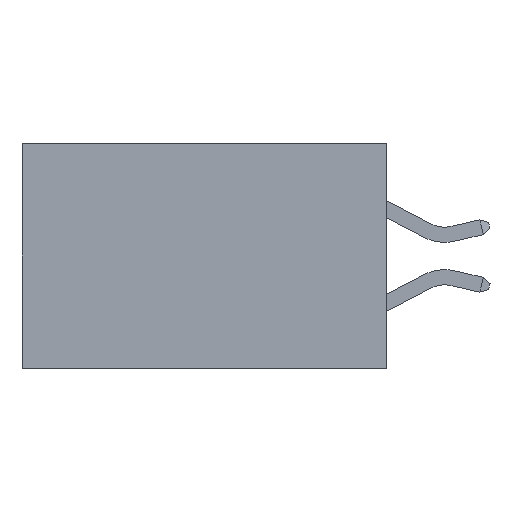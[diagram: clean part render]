
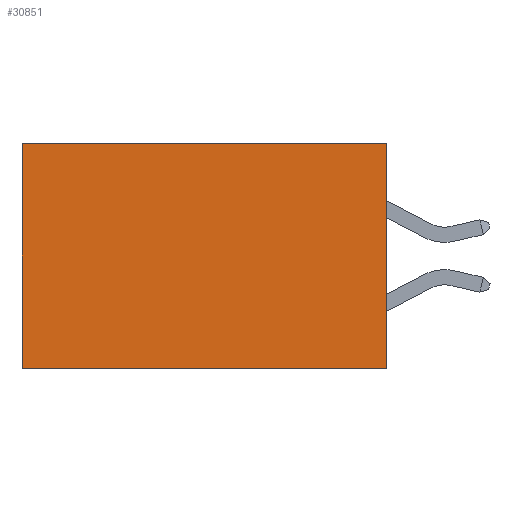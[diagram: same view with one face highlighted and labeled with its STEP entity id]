
A CAD part, left-side view. The second image highlights one B-rep face of the part: STEP entity #30851.
In plain terms, the highlighted planar face has unit normal (-1, 0, 0).
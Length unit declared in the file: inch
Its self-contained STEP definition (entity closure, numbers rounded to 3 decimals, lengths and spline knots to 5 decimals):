
#298 = DIRECTION ( 'NONE',  ( 0., 1., 0. ) ) ;
#1716 = LINE ( 'NONE', #13113, #17820 ) ;
#1743 = VERTEX_POINT ( 'NONE', #19567 ) ;
#1802 = FACE_OUTER_BOUND ( 'NONE', #3720, .T. ) ;
#3399 = CARTESIAN_POINT ( 'NONE',  ( 0.298, 0., 0. ) ) ;
#3720 = EDGE_LOOP ( 'NONE', ( #17352, #19211, #10265, #28102 ) ) ;
#4675 = VECTOR ( 'NONE', #298, 39.37008 ) ;
#5066 = EDGE_CURVE ( 'NONE', #1743, #6829, #15802, .T. ) ;
#5516 = CARTESIAN_POINT ( 'NONE',  ( 0.298, 0., 0. ) ) ;
#5920 = VERTEX_POINT ( 'NONE', #29874 ) ;
#6471 = VECTOR ( 'NONE', #28961, 39.37008 ) ;
#6829 = VERTEX_POINT ( 'NONE', #20515 ) ;
#10265 = ORIENTED_EDGE ( 'NONE', *, *, #27786, .F. ) ;
#10285 = LINE ( 'NONE', #19204, #6471 ) ;
#11252 = CARTESIAN_POINT ( 'NONE',  ( 0.298, 0., -0.37 ) ) ;
#12782 = PLANE ( 'NONE',  #29883 ) ;
#13113 = CARTESIAN_POINT ( 'NONE',  ( 0.298, 0., 0. ) ) ;
#13757 = VERTEX_POINT ( 'NONE', #11252 ) ;
#15802 = LINE ( 'NONE', #5516, #29763 ) ;
#17352 = ORIENTED_EDGE ( 'NONE', *, *, #29684, .T. ) ;
#17820 = VECTOR ( 'NONE', #20658, 39.37008 ) ;
#19204 = CARTESIAN_POINT ( 'NONE',  ( 0.298, 0.6, 0. ) ) ;
#19211 = ORIENTED_EDGE ( 'NONE', *, *, #22162, .F. ) ;
#19567 = CARTESIAN_POINT ( 'NONE',  ( 0.298, 0., 0. ) ) ;
#19731 = CARTESIAN_POINT ( 'NONE',  ( 0.298, 0., -0.37 ) ) ;
#20515 = CARTESIAN_POINT ( 'NONE',  ( 0.298, 0.6, 0. ) ) ;
#20658 = DIRECTION ( 'NONE',  ( 0., 0., -1. ) ) ;
#22162 = EDGE_CURVE ( 'NONE', #13757, #5920, #27351, .T. ) ;
#22834 = DIRECTION ( 'NONE',  ( 1., 0., 0. ) ) ;
#25622 = DIRECTION ( 'NONE',  ( 0., 0., -1. ) ) ;
#27351 = LINE ( 'NONE', #19731, #4675 ) ;
#27682 = DIRECTION ( 'NONE',  ( 0., 1., 0. ) ) ;
#27786 = EDGE_CURVE ( 'NONE', #1743, #13757, #1716, .T. ) ;
#28102 = ORIENTED_EDGE ( 'NONE', *, *, #5066, .T. ) ;
#28961 = DIRECTION ( 'NONE',  ( 0., 0., -1. ) ) ;
#29684 = EDGE_CURVE ( 'NONE', #6829, #5920, #10285, .T. ) ;
#29763 = VECTOR ( 'NONE', #27682, 39.37008 ) ;
#29874 = CARTESIAN_POINT ( 'NONE',  ( 0.298, 0.6, -0.37 ) ) ;
#29883 = AXIS2_PLACEMENT_3D ( 'NONE', #3399, #22834, #25622 ) ;
#30851 = ADVANCED_FACE ( 'NONE', ( #1802 ), #12782, .F. ) ;
